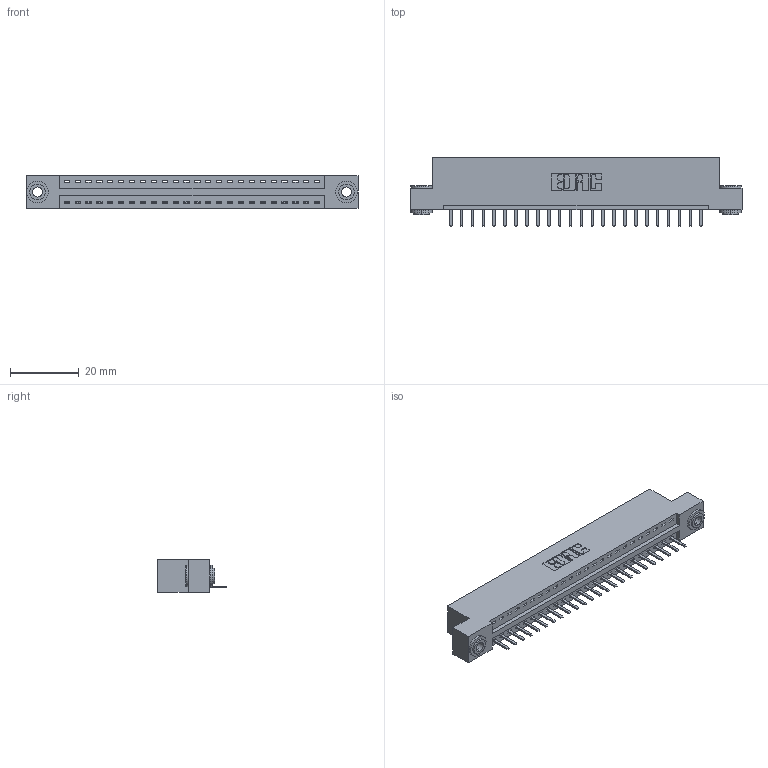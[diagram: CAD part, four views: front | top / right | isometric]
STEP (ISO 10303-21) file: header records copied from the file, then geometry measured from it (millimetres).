
FILE_DESCRIPTION (( 'STEP AP203' ), '1' );
FILE_NAME ('396-024-520-103.STEP', '2019-10-27T05:33:03', ( '' ), ( '' ), 'SwSTEP 2.0', 'SolidWorks 2016', '' );
FILE_SCHEMA (( 'CONFIG_CONTROL_DESIGN' ));
Length unit declared in the file: inch
Products named in the file (4): 345-292-001_345-293-120; 396-024-520-103; 346 Part_Flush Mounting Lugs - 0.156 Dia-TH; 345-250-002_345-250-002-102
Assembly tree (27 placements, depth 2):
  396-024-520-103
    346 Part_Flush Mounting Lugs - 0.156 Dia-TH
    345-292-001_345-293-120  x24
    345-250-002_345-250-002-102  x2
Bounding box: 96.77 x 20.02 x 9.4 mm (x, y, z)
Volume: 9089.8 mm3; surface area: 11155.5 mm2
Topology: 27 solids, 27 shells, 1648 faces, 4821 edges, 3146 vertices
Faces by surface type: plane 1094, cylinder 546, cone 8
Entity records: 18082 total; most frequent: CARTESIAN_POINT 3095, ORIENTED_EDGE 3034, DIRECTION 2771, EDGE_CURVE 1517, VECTOR 1261, LINE 1261, VERTEX_POINT 1006, AXIS2_PLACEMENT_3D 755
